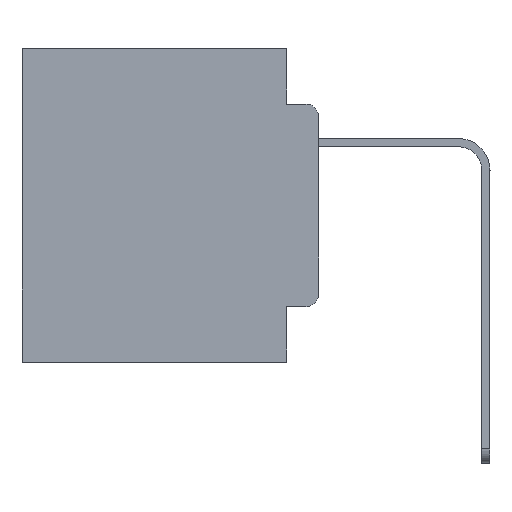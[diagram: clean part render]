
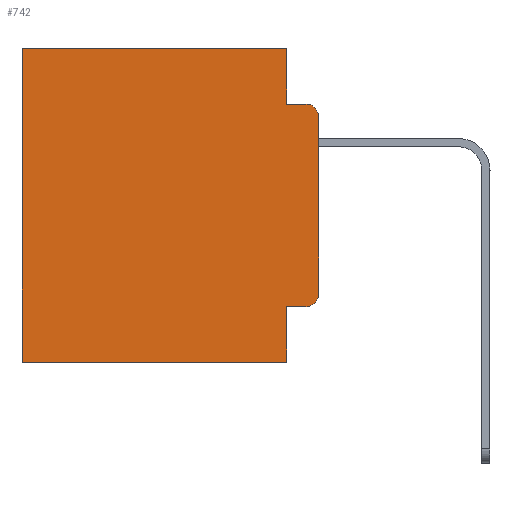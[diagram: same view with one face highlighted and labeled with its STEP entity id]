
A CAD part, left-side view. The second image highlights one B-rep face of the part: STEP entity #742.
In plain terms, the highlighted planar face has unit normal (-1, 0, 0).
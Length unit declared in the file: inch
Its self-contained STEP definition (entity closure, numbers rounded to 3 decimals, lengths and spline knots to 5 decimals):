
#742 = ADVANCED_FACE ( 'NONE', ( #13849 ), #14608, .F. ) ;
#1379 = EDGE_CURVE ( 'NONE', #16608, #10368, #6232, .T. ) ;
#1631 = VERTEX_POINT ( 'NONE', #19968 ) ;
#1658 = VECTOR ( 'NONE', #20181, 39.37008 ) ;
#1730 = CARTESIAN_POINT ( 'NONE',  ( 0.298, 0., 0. ) ) ;
#2611 = VECTOR ( 'NONE', #21956, 39.37008 ) ;
#2796 = VECTOR ( 'NONE', #19012, 39.37008 ) ;
#3622 = CARTESIAN_POINT ( 'NONE',  ( 0.298, 0.051, -0.5 ) ) ;
#3847 = CIRCLE ( 'NONE', #6623, 0.02 ) ;
#4149 = CARTESIAN_POINT ( 'NONE',  ( 0.298, 0., -0.5 ) ) ;
#4476 = ORIENTED_EDGE ( 'NONE', *, *, #14471, .F. ) ;
#5136 = ORIENTED_EDGE ( 'NONE', *, *, #21377, .T. ) ;
#5922 = CARTESIAN_POINT ( 'NONE',  ( 0.298, 0., 0. ) ) ;
#6232 = LINE ( 'NONE', #23608, #2796 ) ;
#6248 = EDGE_CURVE ( 'NONE', #19380, #20025, #12875, .T. ) ;
#6421 = ORIENTED_EDGE ( 'NONE', *, *, #1379, .F. ) ;
#6623 = AXIS2_PLACEMENT_3D ( 'NONE', #9386, #26612, #13512 ) ;
#6755 = EDGE_CURVE ( 'NONE', #14184, #20025, #8342, .T. ) ;
#6861 = CIRCLE ( 'NONE', #7973, 0.02 ) ;
#7357 = VECTOR ( 'NONE', #28363, 39.37008 ) ;
#7624 = CARTESIAN_POINT ( 'NONE',  ( 0.298, 0.051, -0.0885 ) ) ;
#7704 = CARTESIAN_POINT ( 'NONE',  ( 0.298, 0., -0.3915 ) ) ;
#7945 = DIRECTION ( 'NONE',  ( 0., 0., -1. ) ) ;
#7973 = AXIS2_PLACEMENT_3D ( 'NONE', #24197, #15549, #19804 ) ;
#8342 = LINE ( 'NONE', #19376, #18349 ) ;
#8515 = CARTESIAN_POINT ( 'NONE',  ( 0.298, 0.02, -0.4115 ) ) ;
#8789 = ORIENTED_EDGE ( 'NONE', *, *, #11334, .F. ) ;
#8806 = ORIENTED_EDGE ( 'NONE', *, *, #27041, .T. ) ;
#8888 = EDGE_CURVE ( 'NONE', #1631, #11528, #6861, .T. ) ;
#9209 = LINE ( 'NONE', #26784, #1658 ) ;
#9386 = CARTESIAN_POINT ( 'NONE',  ( 0.298, 0.02, -0.3915 ) ) ;
#9522 = CARTESIAN_POINT ( 'NONE',  ( 0.298, 0.02, -0.0885 ) ) ;
#10174 = DIRECTION ( 'NONE',  ( 0., 1., 0. ) ) ;
#10368 = VERTEX_POINT ( 'NONE', #7624 ) ;
#11061 = CARTESIAN_POINT ( 'NONE',  ( 0.298, 0.473, 0. ) ) ;
#11334 = EDGE_CURVE ( 'NONE', #10368, #11528, #16733, .T. ) ;
#11528 = VERTEX_POINT ( 'NONE', #9522 ) ;
#12204 = VECTOR ( 'NONE', #15243, 39.37008 ) ;
#12824 = LINE ( 'NONE', #1730, #7357 ) ;
#12875 = LINE ( 'NONE', #4149, #12204 ) ;
#13512 = DIRECTION ( 'NONE',  ( 0., 0., -1. ) ) ;
#13849 = FACE_OUTER_BOUND ( 'NONE', #26915, .T. ) ;
#14184 = VERTEX_POINT ( 'NONE', #11061 ) ;
#14408 = DIRECTION ( 'NONE',  ( 0., 0., -1. ) ) ;
#14471 = EDGE_CURVE ( 'NONE', #15969, #19380, #22492, .T. ) ;
#14519 = VECTOR ( 'NONE', #10174, 39.37008 ) ;
#14608 = PLANE ( 'NONE',  #18339 ) ;
#14650 = CARTESIAN_POINT ( 'NONE',  ( 0.298, 0.473, -0.5 ) ) ;
#15243 = DIRECTION ( 'NONE',  ( 0., 1., 0. ) ) ;
#15511 = ORIENTED_EDGE ( 'NONE', *, *, #24200, .F. ) ;
#15549 = DIRECTION ( 'NONE',  ( -1., 0., 0. ) ) ;
#15912 = LINE ( 'NONE', #21446, #14519 ) ;
#15969 = VERTEX_POINT ( 'NONE', #24151 ) ;
#16608 = VERTEX_POINT ( 'NONE', #28221 ) ;
#16733 = LINE ( 'NONE', #24257, #2611 ) ;
#16989 = VERTEX_POINT ( 'NONE', #7704 ) ;
#17360 = VECTOR ( 'NONE', #7945, 39.37008 ) ;
#18339 = AXIS2_PLACEMENT_3D ( 'NONE', #5922, #21358, #14408 ) ;
#18349 = VECTOR ( 'NONE', #28099, 39.37008 ) ;
#19012 = DIRECTION ( 'NONE',  ( 0., 0., -1. ) ) ;
#19319 = ORIENTED_EDGE ( 'NONE', *, *, #6248, .F. ) ;
#19376 = CARTESIAN_POINT ( 'NONE',  ( 0.298, 0.473, 0. ) ) ;
#19380 = VERTEX_POINT ( 'NONE', #3622 ) ;
#19804 = DIRECTION ( 'NONE',  ( 0., 0., -1. ) ) ;
#19968 = CARTESIAN_POINT ( 'NONE',  ( 0.298, 0., -0.1085 ) ) ;
#20025 = VERTEX_POINT ( 'NONE', #14650 ) ;
#20181 = DIRECTION ( 'NONE',  ( 0., -1., 0. ) ) ;
#20283 = ORIENTED_EDGE ( 'NONE', *, *, #25413, .T. ) ;
#21358 = DIRECTION ( 'NONE',  ( 1., 0., 0. ) ) ;
#21377 = EDGE_CURVE ( 'NONE', #15969, #23058, #9209, .T. ) ;
#21446 = CARTESIAN_POINT ( 'NONE',  ( 0.298, 0., 0. ) ) ;
#21956 = DIRECTION ( 'NONE',  ( 0., -1., 0. ) ) ;
#22250 = ORIENTED_EDGE ( 'NONE', *, *, #8888, .T. ) ;
#22492 = LINE ( 'NONE', #27783, #17360 ) ;
#23058 = VERTEX_POINT ( 'NONE', #8515 ) ;
#23608 = CARTESIAN_POINT ( 'NONE',  ( 0.298, 0.051, 0. ) ) ;
#23912 = ORIENTED_EDGE ( 'NONE', *, *, #6755, .T. ) ;
#24151 = CARTESIAN_POINT ( 'NONE',  ( 0.298, 0.051, -0.4115 ) ) ;
#24197 = CARTESIAN_POINT ( 'NONE',  ( 0.298, 0.02, -0.1085 ) ) ;
#24200 = EDGE_CURVE ( 'NONE', #1631, #16989, #12824, .T. ) ;
#24257 = CARTESIAN_POINT ( 'NONE',  ( 0.298, 0.051, -0.0885 ) ) ;
#25413 = EDGE_CURVE ( 'NONE', #23058, #16989, #3847, .T. ) ;
#26612 = DIRECTION ( 'NONE',  ( -1., 0., 0. ) ) ;
#26784 = CARTESIAN_POINT ( 'NONE',  ( 0.298, 0.051, -0.4115 ) ) ;
#26915 = EDGE_LOOP ( 'NONE', ( #15511, #22250, #8789, #6421, #8806, #23912, #19319, #4476, #5136, #20283 ) ) ;
#27041 = EDGE_CURVE ( 'NONE', #16608, #14184, #15912, .T. ) ;
#27783 = CARTESIAN_POINT ( 'NONE',  ( 0.298, 0.051, 0. ) ) ;
#28099 = DIRECTION ( 'NONE',  ( 0., 0., -1. ) ) ;
#28221 = CARTESIAN_POINT ( 'NONE',  ( 0.298, 0.051, 0. ) ) ;
#28363 = DIRECTION ( 'NONE',  ( 0., 0., -1. ) ) ;
